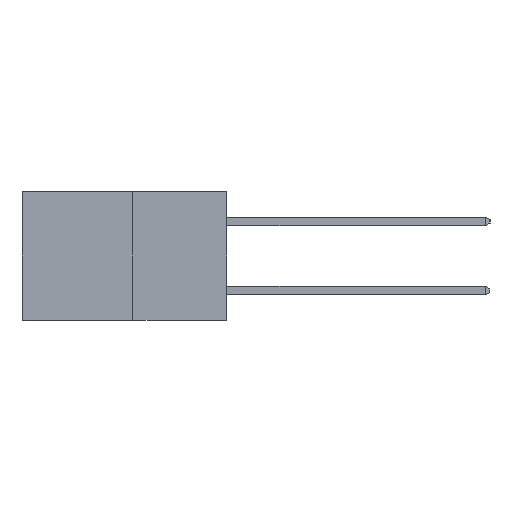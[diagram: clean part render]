
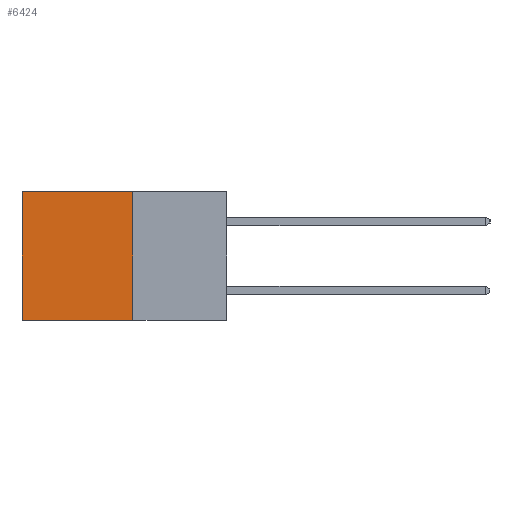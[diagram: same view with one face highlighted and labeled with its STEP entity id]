
A CAD part, left-side view. The second image highlights one B-rep face of the part: STEP entity #6424.
In plain terms, the highlighted planar face has unit normal (-1, 0, 0).
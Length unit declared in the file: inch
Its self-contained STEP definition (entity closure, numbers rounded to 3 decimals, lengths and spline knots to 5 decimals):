
#70 = CARTESIAN_POINT ( 'NONE',  ( 0.277, 0.27, -0.37 ) ) ;
#674 = DIRECTION ( 'NONE',  ( 1., 0., 0. ) ) ;
#1158 = CARTESIAN_POINT ( 'NONE',  ( 0.277, 0.27, -0.37 ) ) ;
#1263 = VERTEX_POINT ( 'NONE', #7531 ) ;
#1289 = EDGE_CURVE ( 'NONE', #4787, #2243, #7039, .T. ) ;
#1313 = DIRECTION ( 'NONE',  ( 0., 1., 0. ) ) ;
#1766 = EDGE_CURVE ( 'NONE', #10536, #1263, #10238, .T. ) ;
#1895 = EDGE_CURVE ( 'NONE', #1263, #2243, #10976, .T. ) ;
#1897 = CARTESIAN_POINT ( 'NONE',  ( 0.277, 0.59, 0. ) ) ;
#1964 = VECTOR ( 'NONE', #10436, 39.37008 ) ;
#2243 = VERTEX_POINT ( 'NONE', #8797 ) ;
#3869 = EDGE_LOOP ( 'NONE', ( #9196, #10588, #3938, #12311 ) ) ;
#3938 = ORIENTED_EDGE ( 'NONE', *, *, #1766, .F. ) ;
#4372 = VECTOR ( 'NONE', #9496, 39.37008 ) ;
#4513 = CARTESIAN_POINT ( 'NONE',  ( 0.277, 0.27, 0. ) ) ;
#4787 = VERTEX_POINT ( 'NONE', #1897 ) ;
#5556 = CARTESIAN_POINT ( 'NONE',  ( 0.277, 0.27, 0. ) ) ;
#6424 = ADVANCED_FACE ( 'NONE', ( #9807 ), #11587, .F. ) ;
#6783 = CARTESIAN_POINT ( 'NONE',  ( 0.277, 0.27, -0.37 ) ) ;
#7039 = LINE ( 'NONE', #9412, #4372 ) ;
#7284 = DIRECTION ( 'NONE',  ( 0., 0., -1. ) ) ;
#7327 = LINE ( 'NONE', #4513, #1964 ) ;
#7330 = VECTOR ( 'NONE', #7284, 39.37008 ) ;
#7528 = EDGE_CURVE ( 'NONE', #10536, #4787, #7327, .T. ) ;
#7531 = CARTESIAN_POINT ( 'NONE',  ( 0.277, 0.27, -0.37 ) ) ;
#7773 = DIRECTION ( 'NONE',  ( 0., 0., -1. ) ) ;
#8385 = VECTOR ( 'NONE', #1313, 39.37008 ) ;
#8797 = CARTESIAN_POINT ( 'NONE',  ( 0.277, 0.59, -0.37 ) ) ;
#9196 = ORIENTED_EDGE ( 'NONE', *, *, #1289, .T. ) ;
#9412 = CARTESIAN_POINT ( 'NONE',  ( 0.277, 0.59, -0.37 ) ) ;
#9496 = DIRECTION ( 'NONE',  ( 0., 0., -1. ) ) ;
#9807 = FACE_OUTER_BOUND ( 'NONE', #3869, .T. ) ;
#10238 = LINE ( 'NONE', #70, #7330 ) ;
#10436 = DIRECTION ( 'NONE',  ( 0., 1., 0. ) ) ;
#10536 = VERTEX_POINT ( 'NONE', #5556 ) ;
#10588 = ORIENTED_EDGE ( 'NONE', *, *, #1895, .F. ) ;
#10976 = LINE ( 'NONE', #1158, #8385 ) ;
#11587 = PLANE ( 'NONE',  #12472 ) ;
#12311 = ORIENTED_EDGE ( 'NONE', *, *, #7528, .T. ) ;
#12472 = AXIS2_PLACEMENT_3D ( 'NONE', #6783, #674, #7773 ) ;
